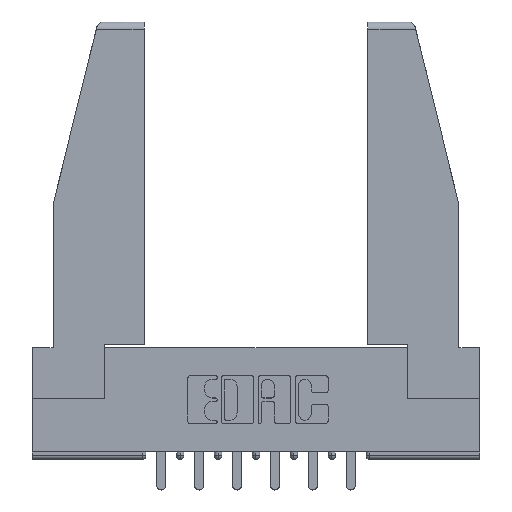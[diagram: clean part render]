
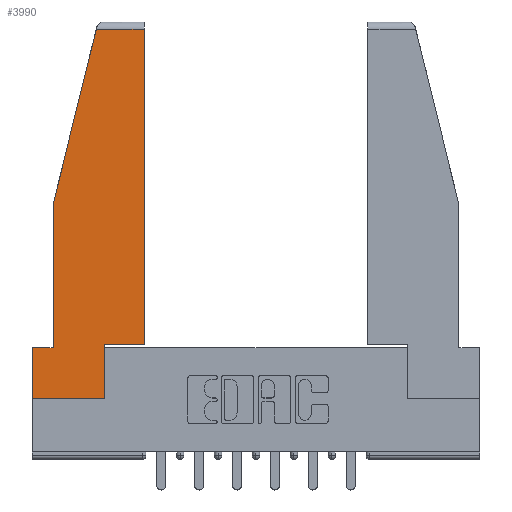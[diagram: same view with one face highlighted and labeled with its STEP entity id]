
A CAD part, top view. The second image highlights one B-rep face of the part: STEP entity #3990.
In plain terms, the highlighted planar face has unit normal (0, 0, 1).
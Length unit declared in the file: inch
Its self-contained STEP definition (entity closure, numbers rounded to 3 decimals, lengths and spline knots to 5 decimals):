
#134 = LINE ( 'NONE', #2789, #5623 ) ;
#166 = CARTESIAN_POINT ( 'NONE',  ( 0., 1.52, 0. ) ) ;
#203 = EDGE_CURVE ( 'NONE', #4136, #3976, #3917, .T. ) ;
#551 = DIRECTION ( 'NONE',  ( 1., 0., 0. ) ) ;
#661 = DIRECTION ( 'NONE',  ( -0.239, -0.971, 0. ) ) ;
#794 = DIRECTION ( 'NONE',  ( -1., 0., 0. ) ) ;
#1140 = ORIENTED_EDGE ( 'NONE', *, *, #203, .T. ) ;
#1723 = VERTEX_POINT ( 'NONE', #10877 ) ;
#1742 = ORIENTED_EDGE ( 'NONE', *, *, #2903, .T. ) ;
#1788 = LINE ( 'NONE', #6143, #4681 ) ;
#1883 = EDGE_CURVE ( 'NONE', #5001, #4136, #6845, .T. ) ;
#2178 = EDGE_CURVE ( 'NONE', #4750, #9757, #7449, .T. ) ;
#2309 = VECTOR ( 'NONE', #7892, 39.37008 ) ;
#2789 = CARTESIAN_POINT ( 'NONE',  ( 0.086, 0.8, 0. ) ) ;
#2903 = EDGE_CURVE ( 'NONE', #3976, #7948, #4327, .T. ) ;
#3023 = FACE_OUTER_BOUND ( 'NONE', #4626, .T. ) ;
#3071 = ORIENTED_EDGE ( 'NONE', *, *, #4037, .T. ) ;
#3465 = CARTESIAN_POINT ( 'NONE',  ( 0.271, 1.55, 0. ) ) ;
#3870 = VECTOR ( 'NONE', #11964, 39.37008 ) ;
#3905 = DIRECTION ( 'NONE',  ( 0., -1., 0. ) ) ;
#3917 = LINE ( 'NONE', #166, #4258 ) ;
#3976 = VERTEX_POINT ( 'NONE', #6882 ) ;
#3990 = ADVANCED_FACE ( 'NONE', ( #3023 ), #12255, .T. ) ;
#4037 = EDGE_CURVE ( 'NONE', #9757, #5001, #11916, .T. ) ;
#4136 = VERTEX_POINT ( 'NONE', #12496 ) ;
#4258 = VECTOR ( 'NONE', #11427, 39.37008 ) ;
#4327 = LINE ( 'NONE', #3465, #9356 ) ;
#4464 = CARTESIAN_POINT ( 'NONE',  ( 0.086, 0.8, 0. ) ) ;
#4616 = EDGE_CURVE ( 'NONE', #9350, #1723, #1788, .T. ) ;
#4626 = EDGE_LOOP ( 'NONE', ( #5013, #1140, #1742, #7314, #5791, #5808, #9877, #12261, #3071 ) ) ;
#4681 = VECTOR ( 'NONE', #794, 39.37008 ) ;
#4750 = VERTEX_POINT ( 'NONE', #9973 ) ;
#4882 = CARTESIAN_POINT ( 'NONE',  ( 0., 0., 0. ) ) ;
#5001 = VERTEX_POINT ( 'NONE', #6633 ) ;
#5013 = ORIENTED_EDGE ( 'NONE', *, *, #1883, .T. ) ;
#5053 = CARTESIAN_POINT ( 'NONE',  ( 0.297, 0.223, 0. ) ) ;
#5096 = LINE ( 'NONE', #9891, #7920 ) ;
#5107 = EDGE_CURVE ( 'NONE', #11333, #4750, #6983, .T. ) ;
#5554 = EDGE_CURVE ( 'NONE', #7948, #9350, #134, .T. ) ;
#5623 = VECTOR ( 'NONE', #3905, 39.37008 ) ;
#5791 = ORIENTED_EDGE ( 'NONE', *, *, #4616, .T. ) ;
#5808 = ORIENTED_EDGE ( 'NONE', *, *, #10604, .T. ) ;
#5885 = CARTESIAN_POINT ( 'NONE',  ( 0.461, 0.223, 0. ) ) ;
#6143 = CARTESIAN_POINT ( 'NONE',  ( 0., 0.21, 0. ) ) ;
#6633 = CARTESIAN_POINT ( 'NONE',  ( 0.461, 0.223, 0. ) ) ;
#6845 = LINE ( 'NONE', #5885, #3870 ) ;
#6882 = CARTESIAN_POINT ( 'NONE',  ( 0.2636, 1.52, 0. ) ) ;
#6983 = LINE ( 'NONE', #4882, #11746 ) ;
#7314 = ORIENTED_EDGE ( 'NONE', *, *, #5554, .T. ) ;
#7449 = LINE ( 'NONE', #9066, #2309 ) ;
#7788 = DIRECTION ( 'NONE',  ( 1., 0., 0. ) ) ;
#7892 = DIRECTION ( 'NONE',  ( 0., 1., 0. ) ) ;
#7920 = VECTOR ( 'NONE', #11639, 39.37008 ) ;
#7924 = DIRECTION ( 'NONE',  ( 1., 0., 0. ) ) ;
#7948 = VERTEX_POINT ( 'NONE', #4464 ) ;
#8911 = AXIS2_PLACEMENT_3D ( 'NONE', #11394, #11355, #551 ) ;
#9066 = CARTESIAN_POINT ( 'NONE',  ( 0.297, 0., 0. ) ) ;
#9350 = VERTEX_POINT ( 'NONE', #11083 ) ;
#9356 = VECTOR ( 'NONE', #661, 39.37008 ) ;
#9548 = VECTOR ( 'NONE', #7924, 39.37008 ) ;
#9757 = VERTEX_POINT ( 'NONE', #10629 ) ;
#9877 = ORIENTED_EDGE ( 'NONE', *, *, #5107, .T. ) ;
#9891 = CARTESIAN_POINT ( 'NONE',  ( 0., 0.21, 0. ) ) ;
#9973 = CARTESIAN_POINT ( 'NONE',  ( 0.297, 0., 0. ) ) ;
#10604 = EDGE_CURVE ( 'NONE', #1723, #11333, #5096, .T. ) ;
#10629 = CARTESIAN_POINT ( 'NONE',  ( 0.297, 0.223, 0. ) ) ;
#10877 = CARTESIAN_POINT ( 'NONE',  ( 0., 0.21, 0. ) ) ;
#10881 = CARTESIAN_POINT ( 'NONE',  ( 0., 0., 0. ) ) ;
#11083 = CARTESIAN_POINT ( 'NONE',  ( 0.086, 0.21, 0. ) ) ;
#11333 = VERTEX_POINT ( 'NONE', #10881 ) ;
#11355 = DIRECTION ( 'NONE',  ( 0., 0., 1. ) ) ;
#11394 = CARTESIAN_POINT ( 'NONE',  ( 0., 0., 0. ) ) ;
#11427 = DIRECTION ( 'NONE',  ( -1., 0., 0. ) ) ;
#11639 = DIRECTION ( 'NONE',  ( 0., -1., 0. ) ) ;
#11746 = VECTOR ( 'NONE', #7788, 39.37008 ) ;
#11916 = LINE ( 'NONE', #5053, #9548 ) ;
#11964 = DIRECTION ( 'NONE',  ( 0., 1., 0. ) ) ;
#12255 = PLANE ( 'NONE',  #8911 ) ;
#12261 = ORIENTED_EDGE ( 'NONE', *, *, #2178, .T. ) ;
#12496 = CARTESIAN_POINT ( 'NONE',  ( 0.461, 1.52, 0. ) ) ;
